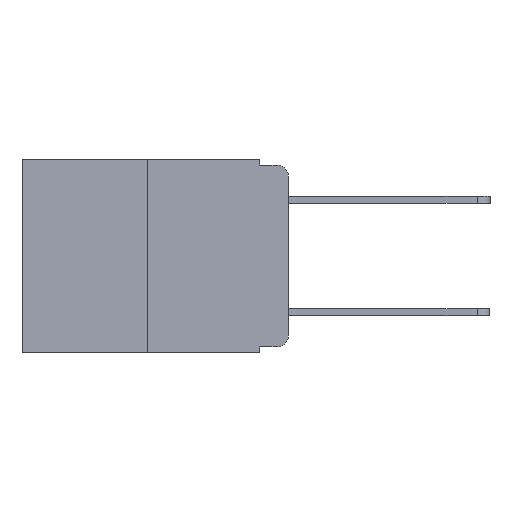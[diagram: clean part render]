
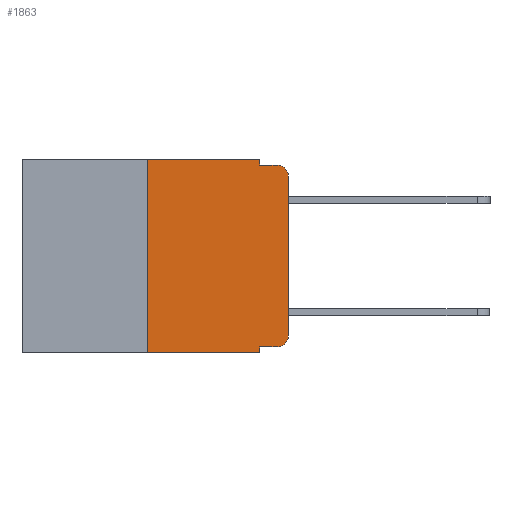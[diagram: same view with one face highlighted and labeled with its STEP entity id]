
A CAD part, left-side view. The second image highlights one B-rep face of the part: STEP entity #1863.
In plain terms, the highlighted planar face has unit normal (-1, 0, 0).
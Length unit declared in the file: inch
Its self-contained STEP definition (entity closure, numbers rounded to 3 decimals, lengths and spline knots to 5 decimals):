
#85 = DIRECTION ( 'NONE',  ( 0., -1., 0. ) ) ;
#100 = DIRECTION ( 'NONE',  ( 0., 0., -1. ) ) ;
#425 = VERTEX_POINT ( 'NONE', #5731 ) ;
#469 = VERTEX_POINT ( 'NONE', #12612 ) ;
#722 = EDGE_CURVE ( 'NONE', #13636, #7379, #13134, .T. ) ;
#872 = CARTESIAN_POINT ( 'NONE',  ( 0., 0.25, 0. ) ) ;
#968 = DIRECTION ( 'NONE',  ( 1., 0., 0. ) ) ;
#1012 = EDGE_CURVE ( 'NONE', #12075, #14297, #4165, .T. ) ;
#1111 = CARTESIAN_POINT ( 'NONE',  ( 0., 0.02, -0.03 ) ) ;
#1154 = DIRECTION ( 'NONE',  ( 0., 0., -1. ) ) ;
#1159 = VECTOR ( 'NONE', #17804, 39.37008 ) ;
#1552 = FACE_OUTER_BOUND ( 'NONE', #8280, .T. ) ;
#1863 = ADVANCED_FACE ( 'NONE', ( #1552 ), #14144, .F. ) ;
#2043 = CARTESIAN_POINT ( 'NONE',  ( 0., 0., 0. ) ) ;
#2068 = CARTESIAN_POINT ( 'NONE',  ( 0., 0.051, -0.333 ) ) ;
#2203 = DIRECTION ( 'NONE',  ( 0., -1., 0. ) ) ;
#2671 = CARTESIAN_POINT ( 'NONE',  ( 0., 0.051, -0.333 ) ) ;
#2733 = VERTEX_POINT ( 'NONE', #15395 ) ;
#2761 = DIRECTION ( 'NONE',  ( 0., 0., -1. ) ) ;
#3491 = LINE ( 'NONE', #872, #11528 ) ;
#3907 = CARTESIAN_POINT ( 'NONE',  ( 0., 0.051, -0.343 ) ) ;
#4165 = CIRCLE ( 'NONE', #8379, 0.02 ) ;
#4194 = CARTESIAN_POINT ( 'NONE',  ( 0., 0.02, -0.313 ) ) ;
#4428 = LINE ( 'NONE', #9977, #15793 ) ;
#4556 = CARTESIAN_POINT ( 'NONE',  ( 0., 0.051, 0. ) ) ;
#4643 = DIRECTION ( 'NONE',  ( 0., 0., -1. ) ) ;
#5067 = VECTOR ( 'NONE', #12617, 39.37008 ) ;
#5152 = EDGE_CURVE ( 'NONE', #2733, #469, #12561, .T. ) ;
#5649 = ORIENTED_EDGE ( 'NONE', *, *, #18921, .T. ) ;
#5694 = ORIENTED_EDGE ( 'NONE', *, *, #12191, .T. ) ;
#5731 = CARTESIAN_POINT ( 'NONE',  ( 0., 0.25, -0.343 ) ) ;
#5940 = DIRECTION ( 'NONE',  ( 0., -1., 0. ) ) ;
#6017 = LINE ( 'NONE', #6738, #1159 ) ;
#6474 = VECTOR ( 'NONE', #5940, 39.37008 ) ;
#6652 = ORIENTED_EDGE ( 'NONE', *, *, #5152, .F. ) ;
#6738 = CARTESIAN_POINT ( 'NONE',  ( 0., 0.473, 0. ) ) ;
#6928 = ORIENTED_EDGE ( 'NONE', *, *, #14543, .F. ) ;
#7028 = VERTEX_POINT ( 'NONE', #4556 ) ;
#7379 = VERTEX_POINT ( 'NONE', #3907 ) ;
#7824 = VECTOR ( 'NONE', #13681, 39.37008 ) ;
#8050 = EDGE_CURVE ( 'NONE', #425, #7379, #4428, .T. ) ;
#8280 = EDGE_LOOP ( 'NONE', ( #5649, #5694, #6652, #6928, #8543, #9232, #9266, #11008, #11882, #14165 ) ) ;
#8379 = AXIS2_PLACEMENT_3D ( 'NONE', #4194, #17926, #4643 ) ;
#8416 = AXIS2_PLACEMENT_3D ( 'NONE', #1111, #11840, #2761 ) ;
#8543 = ORIENTED_EDGE ( 'NONE', *, *, #11860, .F. ) ;
#8662 = LINE ( 'NONE', #2043, #5067 ) ;
#8846 = VECTOR ( 'NONE', #85, 39.37008 ) ;
#9232 = ORIENTED_EDGE ( 'NONE', *, *, #10890, .F. ) ;
#9266 = ORIENTED_EDGE ( 'NONE', *, *, #8050, .T. ) ;
#9615 = CARTESIAN_POINT ( 'NONE',  ( 0., 0.051, -0.01 ) ) ;
#9679 = CARTESIAN_POINT ( 'NONE',  ( 0., 0., -0.03 ) ) ;
#9736 = VERTEX_POINT ( 'NONE', #10226 ) ;
#9977 = CARTESIAN_POINT ( 'NONE',  ( 0., 0.473, -0.343 ) ) ;
#10226 = CARTESIAN_POINT ( 'NONE',  ( 0., 0.25, 0. ) ) ;
#10250 = DIRECTION ( 'NONE',  ( 0., 0., 1. ) ) ;
#10394 = LINE ( 'NONE', #2671, #6474 ) ;
#10588 = CARTESIAN_POINT ( 'NONE',  ( 0., 0., -0.313 ) ) ;
#10890 = EDGE_CURVE ( 'NONE', #425, #9736, #3491, .T. ) ;
#11008 = ORIENTED_EDGE ( 'NONE', *, *, #722, .F. ) ;
#11528 = VECTOR ( 'NONE', #10250, 39.37008 ) ;
#11840 = DIRECTION ( 'NONE',  ( -1., 0., 0. ) ) ;
#11860 = EDGE_CURVE ( 'NONE', #9736, #7028, #6017, .T. ) ;
#11882 = ORIENTED_EDGE ( 'NONE', *, *, #13150, .T. ) ;
#12075 = VERTEX_POINT ( 'NONE', #13030 ) ;
#12191 = EDGE_CURVE ( 'NONE', #14562, #469, #17981, .T. ) ;
#12351 = CARTESIAN_POINT ( 'NONE',  ( 0., 0.473, 0. ) ) ;
#12561 = LINE ( 'NONE', #9615, #8846 ) ;
#12612 = CARTESIAN_POINT ( 'NONE',  ( 0., 0.02, -0.01 ) ) ;
#12617 = DIRECTION ( 'NONE',  ( 0., 0., 1. ) ) ;
#13030 = CARTESIAN_POINT ( 'NONE',  ( 0., 0.02, -0.333 ) ) ;
#13134 = LINE ( 'NONE', #18249, #16645 ) ;
#13150 = EDGE_CURVE ( 'NONE', #13636, #12075, #10394, .T. ) ;
#13636 = VERTEX_POINT ( 'NONE', #2068 ) ;
#13681 = DIRECTION ( 'NONE',  ( 0., 0., -1. ) ) ;
#13734 = CARTESIAN_POINT ( 'NONE',  ( 0., 0.051, 0. ) ) ;
#14144 = PLANE ( 'NONE',  #18347 ) ;
#14165 = ORIENTED_EDGE ( 'NONE', *, *, #1012, .T. ) ;
#14297 = VERTEX_POINT ( 'NONE', #10588 ) ;
#14543 = EDGE_CURVE ( 'NONE', #7028, #2733, #15596, .T. ) ;
#14562 = VERTEX_POINT ( 'NONE', #9679 ) ;
#15395 = CARTESIAN_POINT ( 'NONE',  ( 0., 0.051, -0.01 ) ) ;
#15596 = LINE ( 'NONE', #13734, #7824 ) ;
#15793 = VECTOR ( 'NONE', #2203, 39.37008 ) ;
#16645 = VECTOR ( 'NONE', #1154, 39.37008 ) ;
#17804 = DIRECTION ( 'NONE',  ( 0., -1., 0. ) ) ;
#17926 = DIRECTION ( 'NONE',  ( -1., 0., 0. ) ) ;
#17981 = CIRCLE ( 'NONE', #8416, 0.02 ) ;
#18249 = CARTESIAN_POINT ( 'NONE',  ( 0., 0.051, 0. ) ) ;
#18347 = AXIS2_PLACEMENT_3D ( 'NONE', #12351, #968, #100 ) ;
#18921 = EDGE_CURVE ( 'NONE', #14297, #14562, #8662, .T. ) ;
